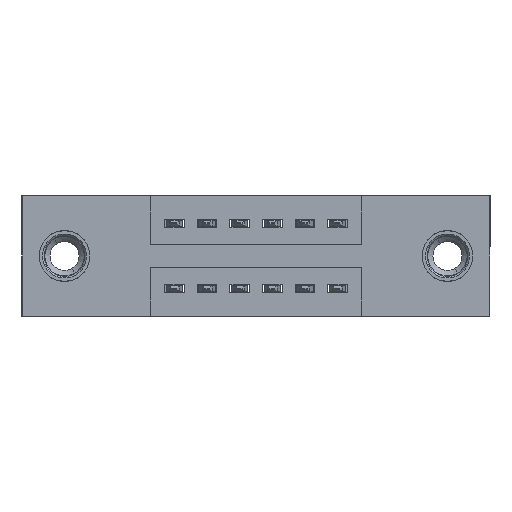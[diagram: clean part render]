
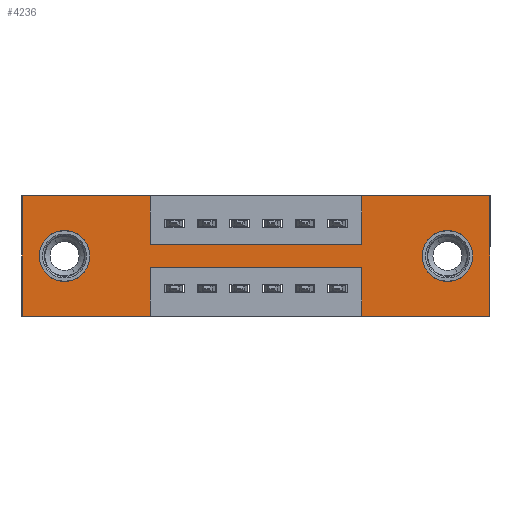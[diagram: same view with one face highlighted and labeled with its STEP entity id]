
A CAD part, front view. The second image highlights one B-rep face of the part: STEP entity #4236.
In plain terms, the highlighted planar face has unit normal (0, -1, 0).
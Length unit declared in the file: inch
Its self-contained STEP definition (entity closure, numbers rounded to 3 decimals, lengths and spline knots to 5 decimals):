
#23 = VERTEX_POINT ( 'NONE', #4599 ) ;
#41 = VECTOR ( 'NONE', #8857, 39.37008 ) ;
#92 = ORIENTED_EDGE ( 'NONE', *, *, #6085, .F. ) ;
#103 = DIRECTION ( 'NONE',  ( 0., 0., -1. ) ) ;
#133 = AXIS2_PLACEMENT_3D ( 'NONE', #1556, #9440, #2735 ) ;
#171 = CARTESIAN_POINT ( 'NONE',  ( 1.0425, 0., -0.22 ) ) ;
#240 = ORIENTED_EDGE ( 'NONE', *, *, #9418, .T. ) ;
#430 = DIRECTION ( 'NONE',  ( 0., 1., 0. ) ) ;
#573 = FACE_BOUND ( 'NONE', #12605, .T. ) ;
#631 = VERTEX_POINT ( 'NONE', #9432 ) ;
#687 = ORIENTED_EDGE ( 'NONE', *, *, #834, .F. ) ;
#761 = CARTESIAN_POINT ( 'NONE',  ( 0.3925, 0., -0.37 ) ) ;
#834 = EDGE_CURVE ( 'NONE', #13164, #4118, #13569, .T. ) ;
#947 = LINE ( 'NONE', #3773, #14331 ) ;
#1418 = VECTOR ( 'NONE', #1831, 39.37008 ) ;
#1449 = CARTESIAN_POINT ( 'NONE',  ( 0.3925, 0., -0.15 ) ) ;
#1506 = CARTESIAN_POINT ( 'NONE',  ( 1.0425, 0., -0.37 ) ) ;
#1510 = ORIENTED_EDGE ( 'NONE', *, *, #4718, .F. ) ;
#1556 = CARTESIAN_POINT ( 'NONE',  ( 0.13, 0., -0.185 ) ) ;
#1724 = CARTESIAN_POINT ( 'NONE',  ( 1.305, 0., -0.107 ) ) ;
#1761 = CARTESIAN_POINT ( 'NONE',  ( 1.0425, 0., -0.15 ) ) ;
#1831 = DIRECTION ( 'NONE',  ( -1., 0., 0. ) ) ;
#2107 = CARTESIAN_POINT ( 'NONE',  ( 0., 0., 0. ) ) ;
#2210 = CARTESIAN_POINT ( 'NONE',  ( 0., 0., 0. ) ) ;
#2219 = VECTOR ( 'NONE', #6436, 39.37008 ) ;
#2383 = CARTESIAN_POINT ( 'NONE',  ( 1.0425, 0., -0.37 ) ) ;
#2624 = LINE ( 'NONE', #761, #2219 ) ;
#2735 = DIRECTION ( 'NONE',  ( 0., 0., 1. ) ) ;
#2761 = CIRCLE ( 'NONE', #133, 0.078 ) ;
#2848 = VERTEX_POINT ( 'NONE', #10920 ) ;
#2961 = EDGE_CURVE ( 'NONE', #631, #14301, #4892, .T. ) ;
#3080 = EDGE_CURVE ( 'NONE', #9397, #11217, #5792, .T. ) ;
#3156 = EDGE_CURVE ( 'NONE', #11140, #631, #10992, .T. ) ;
#3467 = EDGE_CURVE ( 'NONE', #23, #9397, #6473, .T. ) ;
#3683 = CARTESIAN_POINT ( 'NONE',  ( 1.0425, 0., 0. ) ) ;
#3773 = CARTESIAN_POINT ( 'NONE',  ( 0., 0., 0. ) ) ;
#3780 = CARTESIAN_POINT ( 'NONE',  ( 1.305, 0., -0.185 ) ) ;
#3809 = EDGE_CURVE ( 'NONE', #13597, #23, #947, .T. ) ;
#4012 = AXIS2_PLACEMENT_3D ( 'NONE', #10232, #6939, #103 ) ;
#4118 = VERTEX_POINT ( 'NONE', #14389 ) ;
#4236 = ADVANCED_FACE ( 'NONE', ( #573, #12503, #9573 ), #13525, .T. ) ;
#4438 = EDGE_LOOP ( 'NONE', ( #4490, #5682 ) ) ;
#4458 = CIRCLE ( 'NONE', #13710, 0.078 ) ;
#4490 = ORIENTED_EDGE ( 'NONE', *, *, #11537, .T. ) ;
#4587 = CARTESIAN_POINT ( 'NONE',  ( 0.3925, 0., -0.22 ) ) ;
#4599 = CARTESIAN_POINT ( 'NONE',  ( 0.3925, 0., 0. ) ) ;
#4718 = EDGE_CURVE ( 'NONE', #8916, #13597, #12492, .T. ) ;
#4734 = ORIENTED_EDGE ( 'NONE', *, *, #2961, .F. ) ;
#4746 = VECTOR ( 'NONE', #10239, 39.37008 ) ;
#4845 = CARTESIAN_POINT ( 'NONE',  ( 0.3925, 0., 0. ) ) ;
#4879 = DIRECTION ( 'NONE',  ( 0., 0., -1. ) ) ;
#4892 = LINE ( 'NONE', #9960, #10470 ) ;
#4937 = DIRECTION ( 'NONE',  ( 1., 0., 0. ) ) ;
#4948 = DIRECTION ( 'NONE',  ( 0., 0., -1. ) ) ;
#5280 = ORIENTED_EDGE ( 'NONE', *, *, #13272, .T. ) ;
#5364 = VECTOR ( 'NONE', #10285, 39.37008 ) ;
#5488 = LINE ( 'NONE', #5683, #14240 ) ;
#5515 = ORIENTED_EDGE ( 'NONE', *, *, #3156, .F. ) ;
#5682 = ORIENTED_EDGE ( 'NONE', *, *, #9435, .T. ) ;
#5683 = CARTESIAN_POINT ( 'NONE',  ( 1.0425, 0., 0. ) ) ;
#5771 = CIRCLE ( 'NONE', #12478, 0.078 ) ;
#5792 = LINE ( 'NONE', #8843, #41 ) ;
#6085 = EDGE_CURVE ( 'NONE', #12540, #13164, #14116, .T. ) ;
#6251 = AXIS2_PLACEMENT_3D ( 'NONE', #6801, #14447, #7925 ) ;
#6436 = DIRECTION ( 'NONE',  ( 0., 0., -1. ) ) ;
#6473 = LINE ( 'NONE', #4845, #13017 ) ;
#6736 = EDGE_LOOP ( 'NONE', ( #9532, #687, #92, #9902, #4734, #5515, #7159, #13430, #8666, #10837, #1510, #13817 ) ) ;
#6801 = CARTESIAN_POINT ( 'NONE',  ( 0.13, 0., -0.185 ) ) ;
#6935 = EDGE_CURVE ( 'NONE', #11217, #11140, #5488, .T. ) ;
#6939 = DIRECTION ( 'NONE',  ( 0., -1., 0. ) ) ;
#7096 = LINE ( 'NONE', #8645, #1418 ) ;
#7159 = ORIENTED_EDGE ( 'NONE', *, *, #6935, .F. ) ;
#7221 = EDGE_CURVE ( 'NONE', #14301, #12540, #8618, .T. ) ;
#7247 = CARTESIAN_POINT ( 'NONE',  ( 1.305, 0., -0.185 ) ) ;
#7312 = CARTESIAN_POINT ( 'NONE',  ( 0.13, 0., -0.107 ) ) ;
#7559 = CARTESIAN_POINT ( 'NONE',  ( 0.13, 0., -0.263 ) ) ;
#7753 = EDGE_CURVE ( 'NONE', #4118, #8513, #2624, .T. ) ;
#7922 = DIRECTION ( 'NONE',  ( 1., 0., 0. ) ) ;
#7925 = DIRECTION ( 'NONE',  ( 0., 0., 1. ) ) ;
#7986 = CARTESIAN_POINT ( 'NONE',  ( 0., 0., 0. ) ) ;
#8148 = CARTESIAN_POINT ( 'NONE',  ( 1.435, 0., -0.37 ) ) ;
#8382 = DIRECTION ( 'NONE',  ( 0., 0., -1. ) ) ;
#8503 = CARTESIAN_POINT ( 'NONE',  ( 0., 0., -0.37 ) ) ;
#8513 = VERTEX_POINT ( 'NONE', #14174 ) ;
#8618 = LINE ( 'NONE', #12856, #14062 ) ;
#8645 = CARTESIAN_POINT ( 'NONE',  ( 0., 0., -0.37 ) ) ;
#8666 = ORIENTED_EDGE ( 'NONE', *, *, #3467, .F. ) ;
#8843 = CARTESIAN_POINT ( 'NONE',  ( 0.3925, 0., -0.15 ) ) ;
#8857 = DIRECTION ( 'NONE',  ( 1., 0., 0. ) ) ;
#8916 = VERTEX_POINT ( 'NONE', #8503 ) ;
#9397 = VERTEX_POINT ( 'NONE', #1449 ) ;
#9418 = EDGE_CURVE ( 'NONE', #10784, #2848, #5771, .T. ) ;
#9432 = CARTESIAN_POINT ( 'NONE',  ( 1.435, 0., 0. ) ) ;
#9435 = EDGE_CURVE ( 'NONE', #12120, #12611, #2761, .T. ) ;
#9440 = DIRECTION ( 'NONE',  ( 0., 1., 0. ) ) ;
#9532 = ORIENTED_EDGE ( 'NONE', *, *, #7753, .F. ) ;
#9560 = VECTOR ( 'NONE', #12204, 39.37008 ) ;
#9573 = FACE_OUTER_BOUND ( 'NONE', #6736, .T. ) ;
#9902 = ORIENTED_EDGE ( 'NONE', *, *, #7221, .F. ) ;
#9948 = DIRECTION ( 'NONE',  ( 0., 0., -1. ) ) ;
#9960 = CARTESIAN_POINT ( 'NONE',  ( 1.435, 0., 0. ) ) ;
#10232 = CARTESIAN_POINT ( 'NONE',  ( 0., 0., -0.37 ) ) ;
#10239 = DIRECTION ( 'NONE',  ( -1., 0., 0. ) ) ;
#10285 = DIRECTION ( 'NONE',  ( 0., 0., 1. ) ) ;
#10470 = VECTOR ( 'NONE', #9948, 39.37008 ) ;
#10784 = VERTEX_POINT ( 'NONE', #1724 ) ;
#10837 = ORIENTED_EDGE ( 'NONE', *, *, #3809, .F. ) ;
#10920 = CARTESIAN_POINT ( 'NONE',  ( 1.305, 0., -0.263 ) ) ;
#10992 = LINE ( 'NONE', #7986, #13208 ) ;
#11140 = VERTEX_POINT ( 'NONE', #3683 ) ;
#11217 = VERTEX_POINT ( 'NONE', #1761 ) ;
#11415 = CIRCLE ( 'NONE', #6251, 0.078 ) ;
#11537 = EDGE_CURVE ( 'NONE', #12611, #12120, #11415, .T. ) ;
#11604 = DIRECTION ( 'NONE',  ( 0., 1., 0. ) ) ;
#12120 = VERTEX_POINT ( 'NONE', #7559 ) ;
#12204 = DIRECTION ( 'NONE',  ( 0., 0., 1. ) ) ;
#12478 = AXIS2_PLACEMENT_3D ( 'NONE', #3780, #11604, #4948 ) ;
#12492 = LINE ( 'NONE', #2107, #9560 ) ;
#12503 = FACE_BOUND ( 'NONE', #4438, .T. ) ;
#12540 = VERTEX_POINT ( 'NONE', #1506 ) ;
#12605 = EDGE_LOOP ( 'NONE', ( #240, #5280 ) ) ;
#12611 = VERTEX_POINT ( 'NONE', #7312 ) ;
#12856 = CARTESIAN_POINT ( 'NONE',  ( 0., 0., -0.37 ) ) ;
#13017 = VECTOR ( 'NONE', #4879, 39.37008 ) ;
#13164 = VERTEX_POINT ( 'NONE', #171 ) ;
#13208 = VECTOR ( 'NONE', #7922, 39.37008 ) ;
#13272 = EDGE_CURVE ( 'NONE', #2848, #10784, #4458, .T. ) ;
#13390 = DIRECTION ( 'NONE',  ( 0., 0., 1. ) ) ;
#13430 = ORIENTED_EDGE ( 'NONE', *, *, #3080, .F. ) ;
#13525 = PLANE ( 'NONE',  #4012 ) ;
#13569 = LINE ( 'NONE', #4587, #4746 ) ;
#13597 = VERTEX_POINT ( 'NONE', #2210 ) ;
#13710 = AXIS2_PLACEMENT_3D ( 'NONE', #7247, #430, #8382 ) ;
#13817 = ORIENTED_EDGE ( 'NONE', *, *, #14040, .F. ) ;
#13931 = DIRECTION ( 'NONE',  ( -1., 0., 0. ) ) ;
#14040 = EDGE_CURVE ( 'NONE', #8513, #8916, #7096, .T. ) ;
#14062 = VECTOR ( 'NONE', #13931, 39.37008 ) ;
#14116 = LINE ( 'NONE', #2383, #5364 ) ;
#14174 = CARTESIAN_POINT ( 'NONE',  ( 0.3925, 0., -0.37 ) ) ;
#14240 = VECTOR ( 'NONE', #13390, 39.37008 ) ;
#14301 = VERTEX_POINT ( 'NONE', #8148 ) ;
#14331 = VECTOR ( 'NONE', #4937, 39.37008 ) ;
#14389 = CARTESIAN_POINT ( 'NONE',  ( 0.3925, 0., -0.22 ) ) ;
#14447 = DIRECTION ( 'NONE',  ( 0., 1., 0. ) ) ;
